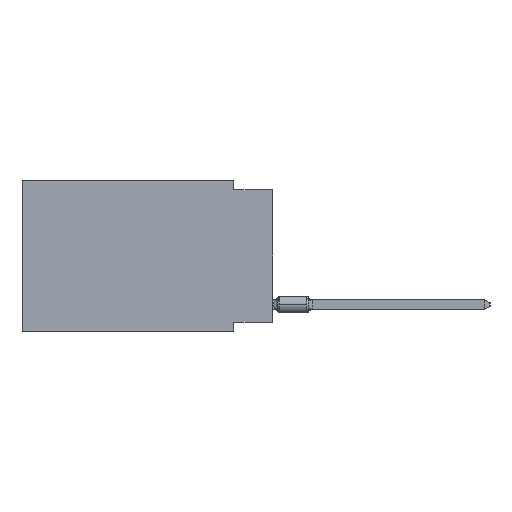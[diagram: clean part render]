
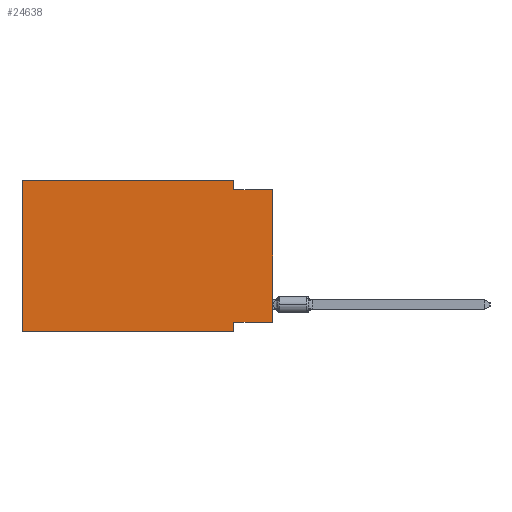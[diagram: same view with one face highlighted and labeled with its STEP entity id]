
A CAD part, left-side view. The second image highlights one B-rep face of the part: STEP entity #24638.
In plain terms, the highlighted planar face has unit normal (-1, 0, 0).
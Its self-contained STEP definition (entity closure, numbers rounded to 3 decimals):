
#132 = CARTESIAN_POINT ( 'NONE',  ( 0., 16.383, -9.906 ) ) ;
#1131 = CARTESIAN_POINT ( 'NONE',  ( 0., 2.54, 0. ) ) ;
#3350 = VERTEX_POINT ( 'NONE', #132 ) ;
#3693 = CARTESIAN_POINT ( 'NONE',  ( 0., 16.383, 0. ) ) ;
#4576 = VERTEX_POINT ( 'NONE', #23550 ) ;
#4871 = EDGE_CURVE ( 'NONE', #14344, #19583, #31335, .T. ) ;
#5381 = ORIENTED_EDGE ( 'NONE', *, *, #19440, .T. ) ;
#6230 = DIRECTION ( 'NONE',  ( 0., -1., 0. ) ) ;
#6482 = CARTESIAN_POINT ( 'NONE',  ( 0., 0., -0.635 ) ) ;
#6980 = LINE ( 'NONE', #33455, #34744 ) ;
#7963 = CARTESIAN_POINT ( 'NONE',  ( 0., 16.383, 0. ) ) ;
#9434 = LINE ( 'NONE', #31709, #29119 ) ;
#9986 = CARTESIAN_POINT ( 'NONE',  ( 0., 16.383, -9.906 ) ) ;
#10037 = EDGE_LOOP ( 'NONE', ( #5381, #33755, #25627, #33862, #24579, #20868, #29826, #26907 ) ) ;
#11425 = VECTOR ( 'NONE', #40794, 1000. ) ;
#11859 = LINE ( 'NONE', #40647, #39858 ) ;
#11957 = DIRECTION ( 'NONE',  ( 0., 1., 0. ) ) ;
#12199 = CARTESIAN_POINT ( 'NONE',  ( 0., 16.383, 0. ) ) ;
#13102 = EDGE_CURVE ( 'NONE', #3350, #4576, #22379, .T. ) ;
#13424 = DIRECTION ( 'NONE',  ( 1., 0., 0. ) ) ;
#13728 = EDGE_CURVE ( 'NONE', #23150, #4576, #6980, .T. ) ;
#14182 = VECTOR ( 'NONE', #15436, 1000. ) ;
#14344 = VERTEX_POINT ( 'NONE', #3693 ) ;
#15436 = DIRECTION ( 'NONE',  ( 0., 0., 1. ) ) ;
#17412 = PLANE ( 'NONE',  #28492 ) ;
#18451 = CARTESIAN_POINT ( 'NONE',  ( 0., 0., -9.271 ) ) ;
#19440 = EDGE_CURVE ( 'NONE', #36096, #38264, #25735, .T. ) ;
#19583 = VERTEX_POINT ( 'NONE', #1131 ) ;
#20868 = ORIENTED_EDGE ( 'NONE', *, *, #13102, .T. ) ;
#22035 = CARTESIAN_POINT ( 'NONE',  ( 0., 2.54, -9.271 ) ) ;
#22379 = LINE ( 'NONE', #9986, #22627 ) ;
#22581 = CARTESIAN_POINT ( 'NONE',  ( 0., 0., 0. ) ) ;
#22627 = VECTOR ( 'NONE', #38346, 1000. ) ;
#22735 = DIRECTION ( 'NONE',  ( 0., 0., 1. ) ) ;
#23150 = VERTEX_POINT ( 'NONE', #22035 ) ;
#23550 = CARTESIAN_POINT ( 'NONE',  ( 0., 2.54, -9.906 ) ) ;
#24516 = VECTOR ( 'NONE', #6230, 1000. ) ;
#24579 = ORIENTED_EDGE ( 'NONE', *, *, #31038, .F. ) ;
#24638 = ADVANCED_FACE ( 'NONE', ( #29609 ), #17412, .F. ) ;
#24884 = DIRECTION ( 'NONE',  ( 0., 0., -1. ) ) ;
#25627 = ORIENTED_EDGE ( 'NONE', *, *, #32268, .F. ) ;
#25735 = LINE ( 'NONE', #22581, #14182 ) ;
#26354 = EDGE_CURVE ( 'NONE', #28906, #38264, #35014, .T. ) ;
#26715 = CARTESIAN_POINT ( 'NONE',  ( 0., 16.383, 0. ) ) ;
#26865 = CARTESIAN_POINT ( 'NONE',  ( 0., 2.54, -0.635 ) ) ;
#26907 = ORIENTED_EDGE ( 'NONE', *, *, #34666, .F. ) ;
#28492 = AXIS2_PLACEMENT_3D ( 'NONE', #7963, #13424, #35897 ) ;
#28906 = VERTEX_POINT ( 'NONE', #26865 ) ;
#29119 = VECTOR ( 'NONE', #11957, 1000. ) ;
#29609 = FACE_OUTER_BOUND ( 'NONE', #10037, .T. ) ;
#29826 = ORIENTED_EDGE ( 'NONE', *, *, #13728, .F. ) ;
#29855 = LINE ( 'NONE', #26715, #36802 ) ;
#31038 = EDGE_CURVE ( 'NONE', #3350, #14344, #29855, .T. ) ;
#31335 = LINE ( 'NONE', #12199, #11425 ) ;
#31456 = CARTESIAN_POINT ( 'NONE',  ( 0., 0., -0.635 ) ) ;
#31709 = CARTESIAN_POINT ( 'NONE',  ( 0., 0., -9.271 ) ) ;
#32268 = EDGE_CURVE ( 'NONE', #19583, #28906, #11859, .T. ) ;
#33455 = CARTESIAN_POINT ( 'NONE',  ( 0., 2.54, -9.906 ) ) ;
#33755 = ORIENTED_EDGE ( 'NONE', *, *, #26354, .F. ) ;
#33862 = ORIENTED_EDGE ( 'NONE', *, *, #4871, .F. ) ;
#34666 = EDGE_CURVE ( 'NONE', #36096, #23150, #9434, .T. ) ;
#34744 = VECTOR ( 'NONE', #39549, 1000. ) ;
#35014 = LINE ( 'NONE', #31456, #24516 ) ;
#35897 = DIRECTION ( 'NONE',  ( 0., 0., -1. ) ) ;
#36096 = VERTEX_POINT ( 'NONE', #18451 ) ;
#36802 = VECTOR ( 'NONE', #22735, 1000. ) ;
#38264 = VERTEX_POINT ( 'NONE', #6482 ) ;
#38346 = DIRECTION ( 'NONE',  ( 0., -1., 0. ) ) ;
#39549 = DIRECTION ( 'NONE',  ( 0., 0., -1. ) ) ;
#39858 = VECTOR ( 'NONE', #24884, 1000. ) ;
#40647 = CARTESIAN_POINT ( 'NONE',  ( 0., 2.54, 0. ) ) ;
#40794 = DIRECTION ( 'NONE',  ( 0., -1., 0. ) ) ;
